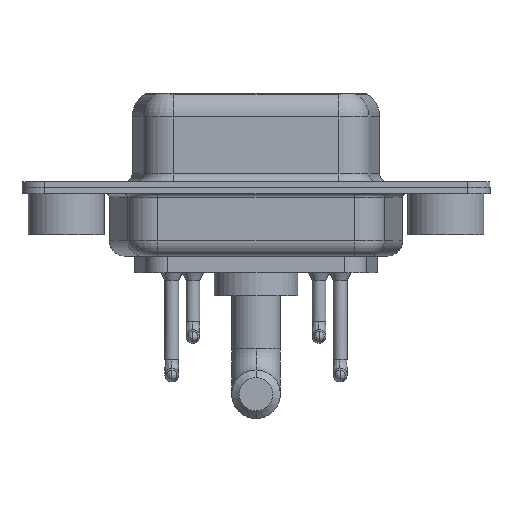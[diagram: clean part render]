
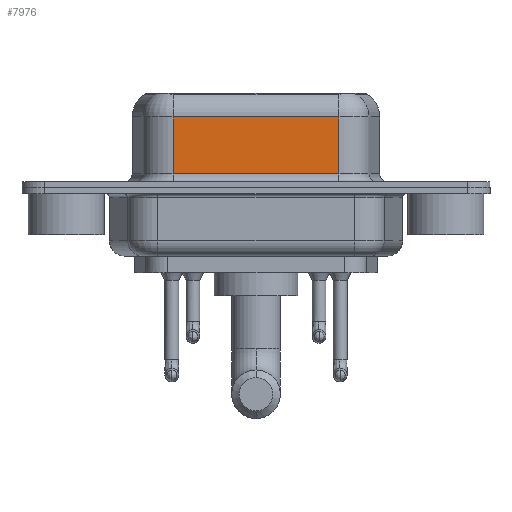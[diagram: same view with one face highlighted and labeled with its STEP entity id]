
A CAD part, front view. The second image highlights one B-rep face of the part: STEP entity #7976.
In plain terms, the highlighted planar face has unit normal (0, -1, 0).
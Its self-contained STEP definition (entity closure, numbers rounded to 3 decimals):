
#554 = DIRECTION ( 'NONE',  ( -1., 0., 0. ) ) ;
#680 = EDGE_CURVE ( 'NONE', #9008, #2652, #5434, .T. ) ;
#1631 = VERTEX_POINT ( 'NONE', #11453 ) ;
#2018 = ORIENTED_EDGE ( 'NONE', *, *, #13044, .T. ) ;
#2364 = VERTEX_POINT ( 'NONE', #12773 ) ;
#2419 = EDGE_CURVE ( 'NONE', #2364, #2652, #5311, .T. ) ;
#2652 = VERTEX_POINT ( 'NONE', #13584 ) ;
#2842 = PLANE ( 'NONE',  #8629 ) ;
#3783 = CARTESIAN_POINT ( 'NONE',  ( 7.038, -3.95, 0.9 ) ) ;
#4805 = ORIENTED_EDGE ( 'NONE', *, *, #2419, .F. ) ;
#5311 = LINE ( 'NONE', #12689, #11810 ) ;
#5434 = LINE ( 'NONE', #14062, #10947 ) ;
#5841 = DIRECTION ( 'NONE',  ( 0., 0., -1. ) ) ;
#6519 = DIRECTION ( 'NONE',  ( 1., 0., 0. ) ) ;
#6627 = DIRECTION ( 'NONE',  ( 0., 1., 0. ) ) ;
#6699 = VECTOR ( 'NONE', #554, 1000. ) ;
#6914 = LINE ( 'NONE', #14528, #6699 ) ;
#7252 = CARTESIAN_POINT ( 'NONE',  ( 7.038, -3.95, 6.4 ) ) ;
#7513 = EDGE_LOOP ( 'NONE', ( #4805, #10071, #2018, #8211 ) ) ;
#7862 = DIRECTION ( 'NONE',  ( 0., 0., -1. ) ) ;
#7976 = ADVANCED_FACE ( 'NONE', ( #9107 ), #2842, .F. ) ;
#8211 = ORIENTED_EDGE ( 'NONE', *, *, #680, .T. ) ;
#8629 = AXIS2_PLACEMENT_3D ( 'NONE', #12930, #6627, #11686 ) ;
#9008 = VERTEX_POINT ( 'NONE', #3783 ) ;
#9107 = FACE_OUTER_BOUND ( 'NONE', #7513, .T. ) ;
#10071 = ORIENTED_EDGE ( 'NONE', *, *, #15681, .T. ) ;
#10947 = VECTOR ( 'NONE', #6519, 1000. ) ;
#11122 = VECTOR ( 'NONE', #5841, 1000. ) ;
#11453 = CARTESIAN_POINT ( 'NONE',  ( 7.038, -3.95, 4.65 ) ) ;
#11686 = DIRECTION ( 'NONE',  ( -1., 0., 0. ) ) ;
#11810 = VECTOR ( 'NONE', #7862, 1000. ) ;
#12689 = CARTESIAN_POINT ( 'NONE',  ( 17.962, -3.95, 6.4 ) ) ;
#12773 = CARTESIAN_POINT ( 'NONE',  ( 17.962, -3.95, 4.65 ) ) ;
#12930 = CARTESIAN_POINT ( 'NONE',  ( 17.962, -3.95, 6.4 ) ) ;
#13044 = EDGE_CURVE ( 'NONE', #1631, #9008, #13634, .T. ) ;
#13584 = CARTESIAN_POINT ( 'NONE',  ( 17.962, -3.95, 0.9 ) ) ;
#13634 = LINE ( 'NONE', #7252, #11122 ) ;
#14062 = CARTESIAN_POINT ( 'NONE',  ( 17.962, -3.95, 0.9 ) ) ;
#14528 = CARTESIAN_POINT ( 'NONE',  ( 17.962, -3.95, 4.65 ) ) ;
#15681 = EDGE_CURVE ( 'NONE', #2364, #1631, #6914, .T. ) ;
